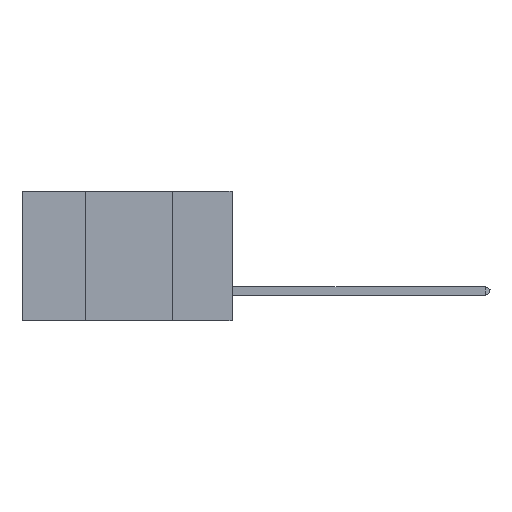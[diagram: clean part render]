
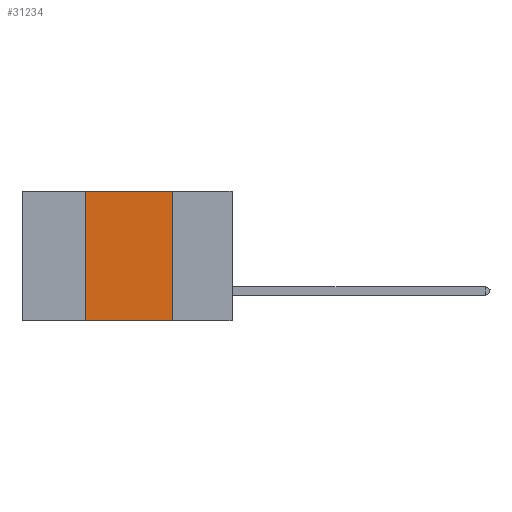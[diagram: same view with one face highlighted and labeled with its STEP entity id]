
A CAD part, left-side view. The second image highlights one B-rep face of the part: STEP entity #31234.
In plain terms, the highlighted planar face has unit normal (-1, 0, 0).
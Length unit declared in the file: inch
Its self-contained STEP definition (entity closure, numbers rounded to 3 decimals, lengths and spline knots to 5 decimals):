
#441 = VERTEX_POINT ( 'NONE', #45045 ) ;
#820 = VECTOR ( 'NONE', #37076, 39.37008 ) ;
#2884 = EDGE_LOOP ( 'NONE', ( #18368, #44933, #29101, #20066 ) ) ;
#3104 = CARTESIAN_POINT ( 'NONE',  ( 0., 0.17, -0.37 ) ) ;
#5013 = CARTESIAN_POINT ( 'NONE',  ( 0., 0.6, 0. ) ) ;
#5462 = VECTOR ( 'NONE', #41927, 39.37008 ) ;
#11139 = VECTOR ( 'NONE', #39878, 39.37008 ) ;
#12370 = FACE_OUTER_BOUND ( 'NONE', #2884, .T. ) ;
#13351 = EDGE_CURVE ( 'NONE', #20644, #441, #26446, .T. ) ;
#13635 = CARTESIAN_POINT ( 'NONE',  ( 0., 0.17, 0. ) ) ;
#14909 = CARTESIAN_POINT ( 'NONE',  ( 0., 0.42, -0.37 ) ) ;
#15109 = CARTESIAN_POINT ( 'NONE',  ( 0., 0.42, 0. ) ) ;
#15638 = VECTOR ( 'NONE', #35663, 39.37008 ) ;
#17343 = VERTEX_POINT ( 'NONE', #14909 ) ;
#17723 = EDGE_CURVE ( 'NONE', #17343, #26723, #42717, .T. ) ;
#18212 = DIRECTION ( 'NONE',  ( 0., 0., -1. ) ) ;
#18368 = ORIENTED_EDGE ( 'NONE', *, *, #39583, .F. ) ;
#18702 = AXIS2_PLACEMENT_3D ( 'NONE', #5013, #20167, #18212 ) ;
#18866 = PLANE ( 'NONE',  #18702 ) ;
#20066 = ORIENTED_EDGE ( 'NONE', *, *, #17723, .T. ) ;
#20167 = DIRECTION ( 'NONE',  ( 1., 0., 0. ) ) ;
#20644 = VERTEX_POINT ( 'NONE', #44815 ) ;
#26446 = LINE ( 'NONE', #35283, #11139 ) ;
#26723 = VERTEX_POINT ( 'NONE', #3104 ) ;
#27487 = EDGE_CURVE ( 'NONE', #17343, #20644, #29770, .T. ) ;
#29101 = ORIENTED_EDGE ( 'NONE', *, *, #27487, .F. ) ;
#29770 = LINE ( 'NONE', #15109, #15638 ) ;
#30040 = CARTESIAN_POINT ( 'NONE',  ( 0., 0.6, -0.37 ) ) ;
#31234 = ADVANCED_FACE ( 'NONE', ( #12370 ), #18866, .F. ) ;
#35283 = CARTESIAN_POINT ( 'NONE',  ( 0., 0.6, 0. ) ) ;
#35663 = DIRECTION ( 'NONE',  ( 0., 0., 1. ) ) ;
#37076 = DIRECTION ( 'NONE',  ( 0., -1., 0. ) ) ;
#39583 = EDGE_CURVE ( 'NONE', #441, #26723, #43006, .T. ) ;
#39878 = DIRECTION ( 'NONE',  ( 0., -1., 0. ) ) ;
#41927 = DIRECTION ( 'NONE',  ( 0., 0., -1. ) ) ;
#42717 = LINE ( 'NONE', #30040, #820 ) ;
#43006 = LINE ( 'NONE', #13635, #5462 ) ;
#44815 = CARTESIAN_POINT ( 'NONE',  ( 0., 0.42, 0. ) ) ;
#44933 = ORIENTED_EDGE ( 'NONE', *, *, #13351, .F. ) ;
#45045 = CARTESIAN_POINT ( 'NONE',  ( 0., 0.17, 0. ) ) ;
